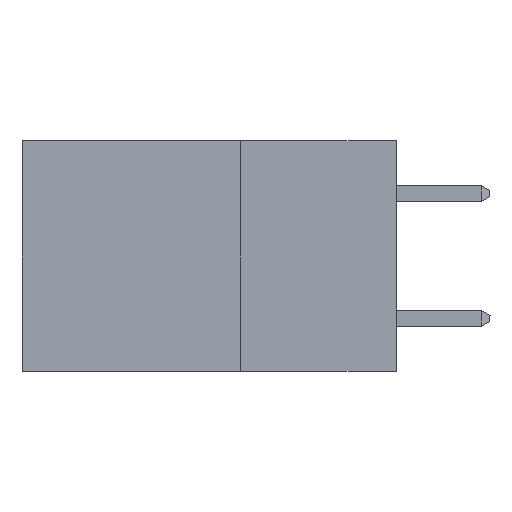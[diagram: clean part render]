
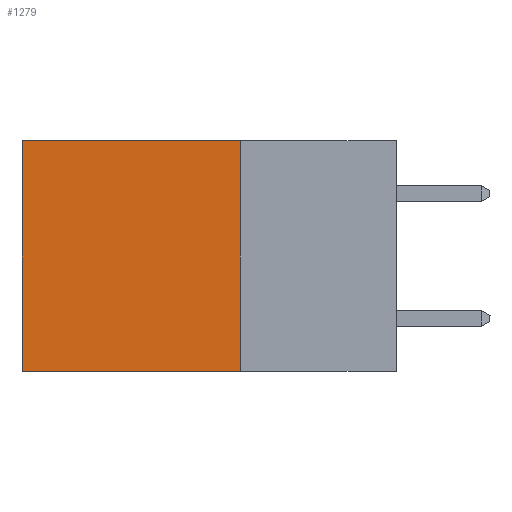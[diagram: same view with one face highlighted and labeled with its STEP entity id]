
A CAD part, left-side view. The second image highlights one B-rep face of the part: STEP entity #1279.
In plain terms, the highlighted planar face has unit normal (-1, 0, 0).
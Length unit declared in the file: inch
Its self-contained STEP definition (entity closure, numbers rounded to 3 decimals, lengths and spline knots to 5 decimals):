
#158 = ORIENTED_EDGE ( 'NONE', *, *, #14544, .F. ) ;
#1057 = VECTOR ( 'NONE', #14872, 39.37008 ) ;
#1112 = EDGE_CURVE ( 'NONE', #13370, #2235, #7523, .T. ) ;
#1279 = ADVANCED_FACE ( 'NONE', ( #9094 ), #12730, .F. ) ;
#2235 = VERTEX_POINT ( 'NONE', #14870 ) ;
#3010 = VERTEX_POINT ( 'NONE', #7395 ) ;
#3365 = CARTESIAN_POINT ( 'NONE',  ( 0.2615, 0.25, 0. ) ) ;
#4268 = LINE ( 'NONE', #11643, #14694 ) ;
#5027 = CARTESIAN_POINT ( 'NONE',  ( 0.2615, 0.6, -0.37 ) ) ;
#5225 = CARTESIAN_POINT ( 'NONE',  ( 0.2615, 0.6, 0. ) ) ;
#5367 = DIRECTION ( 'NONE',  ( 0., 1., 0. ) ) ;
#5383 = ORIENTED_EDGE ( 'NONE', *, *, #1112, .T. ) ;
#5639 = EDGE_CURVE ( 'NONE', #8478, #3010, #7923, .T. ) ;
#7395 = CARTESIAN_POINT ( 'NONE',  ( 0.2615, 0.25, -0.37 ) ) ;
#7523 = LINE ( 'NONE', #5027, #10483 ) ;
#7673 = EDGE_LOOP ( 'NONE', ( #5383, #158, #14798, #7770 ) ) ;
#7770 = ORIENTED_EDGE ( 'NONE', *, *, #11065, .T. ) ;
#7923 = LINE ( 'NONE', #14897, #1057 ) ;
#8125 = DIRECTION ( 'NONE',  ( 0., 1., 0. ) ) ;
#8211 = AXIS2_PLACEMENT_3D ( 'NONE', #12623, #12498, #12464 ) ;
#8478 = VERTEX_POINT ( 'NONE', #3365 ) ;
#8892 = VECTOR ( 'NONE', #8125, 39.37008 ) ;
#8919 = CARTESIAN_POINT ( 'NONE',  ( 0.2615, 0.25, 0. ) ) ;
#9094 = FACE_OUTER_BOUND ( 'NONE', #7673, .T. ) ;
#10483 = VECTOR ( 'NONE', #16224, 39.37008 ) ;
#11065 = EDGE_CURVE ( 'NONE', #8478, #13370, #15142, .T. ) ;
#11643 = CARTESIAN_POINT ( 'NONE',  ( 0.2615, 0.25, -0.37 ) ) ;
#12464 = DIRECTION ( 'NONE',  ( 0., 0., -1. ) ) ;
#12498 = DIRECTION ( 'NONE',  ( 1., 0., 0. ) ) ;
#12623 = CARTESIAN_POINT ( 'NONE',  ( 0.2615, 0.25, -0.37 ) ) ;
#12730 = PLANE ( 'NONE',  #8211 ) ;
#13370 = VERTEX_POINT ( 'NONE', #5225 ) ;
#14544 = EDGE_CURVE ( 'NONE', #3010, #2235, #4268, .T. ) ;
#14694 = VECTOR ( 'NONE', #5367, 39.37008 ) ;
#14798 = ORIENTED_EDGE ( 'NONE', *, *, #5639, .F. ) ;
#14870 = CARTESIAN_POINT ( 'NONE',  ( 0.2615, 0.6, -0.37 ) ) ;
#14872 = DIRECTION ( 'NONE',  ( 0., 0., -1. ) ) ;
#14897 = CARTESIAN_POINT ( 'NONE',  ( 0.2615, 0.25, -0.37 ) ) ;
#15142 = LINE ( 'NONE', #8919, #8892 ) ;
#16224 = DIRECTION ( 'NONE',  ( 0., 0., -1. ) ) ;
